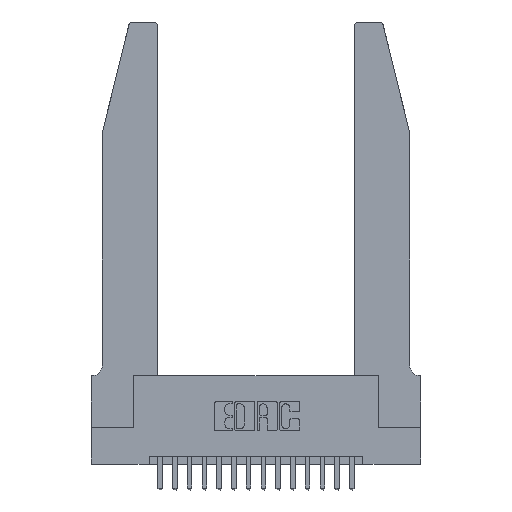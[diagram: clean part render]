
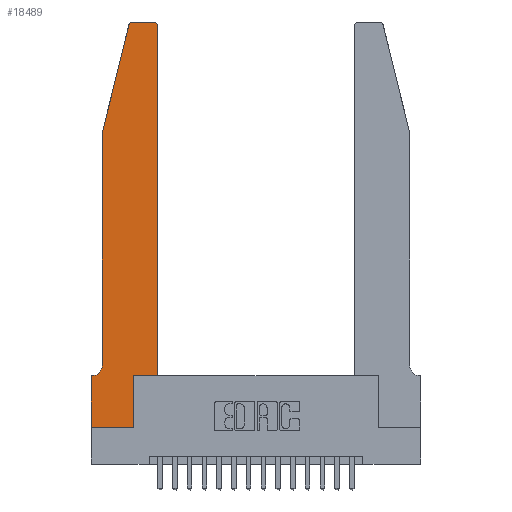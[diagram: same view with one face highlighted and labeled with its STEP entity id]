
A CAD part, top view. The second image highlights one B-rep face of the part: STEP entity #18489.
In plain terms, the highlighted planar face has unit normal (0, 0, 1).
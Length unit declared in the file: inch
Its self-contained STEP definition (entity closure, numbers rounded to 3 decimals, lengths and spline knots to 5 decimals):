
#10 = CARTESIAN_POINT ( 'NONE',  ( 0.2865, 0.35, 0.37 ) ) ;
#383 = ORIENTED_EDGE ( 'NONE', *, *, #14415, .T. ) ;
#557 = DIRECTION ( 'NONE',  ( 0., -1., 0. ) ) ;
#565 = EDGE_CURVE ( 'NONE', #1459, #2175, #1301, .T. ) ;
#657 = CARTESIAN_POINT ( 'NONE',  ( 0.25487, 2.72718, 0.37 ) ) ;
#998 = CARTESIAN_POINT ( 'NONE',  ( 0.0055, 0.35, 0.37 ) ) ;
#1287 = VERTEX_POINT ( 'NONE', #17389 ) ;
#1301 = LINE ( 'NONE', #3186, #13107 ) ;
#1307 = CARTESIAN_POINT ( 'NONE',  ( 0.284, 2.72, 0.37 ) ) ;
#1415 = DIRECTION ( 'NONE',  ( 0., 1., 0. ) ) ;
#1459 = VERTEX_POINT ( 'NONE', #657 ) ;
#1887 = ORIENTED_EDGE ( 'NONE', *, *, #7850, .T. ) ;
#1935 = LINE ( 'NONE', #6139, #17529 ) ;
#2174 = EDGE_CURVE ( 'NONE', #6548, #7849, #13315, .T. ) ;
#2175 = VERTEX_POINT ( 'NONE', #17664 ) ;
#2743 = EDGE_CURVE ( 'NONE', #13909, #16996, #7911, .T. ) ;
#2886 = LINE ( 'NONE', #12141, #7076 ) ;
#2912 = DIRECTION ( 'NONE',  ( 1., 0., 0. ) ) ;
#3186 = CARTESIAN_POINT ( 'NONE',  ( 0.0755, 2., 0.37 ) ) ;
#3540 = AXIS2_PLACEMENT_3D ( 'NONE', #13201, #4054, #14650 ) ;
#3623 = EDGE_CURVE ( 'NONE', #14515, #13909, #11487, .T. ) ;
#3735 = DIRECTION ( 'NONE',  ( 0., 0., -1. ) ) ;
#3985 = CARTESIAN_POINT ( 'NONE',  ( 0.284, 2.75, 0.37 ) ) ;
#4054 = DIRECTION ( 'NONE',  ( 0., 0., 1. ) ) ;
#4196 = VECTOR ( 'NONE', #557, 39.37008 ) ;
#4371 = VERTEX_POINT ( 'NONE', #19359 ) ;
#4675 = ORIENTED_EDGE ( 'NONE', *, *, #2743, .T. ) ;
#4690 = EDGE_CURVE ( 'NONE', #1287, #6548, #13777, .T. ) ;
#5369 = CARTESIAN_POINT ( 'NONE',  ( 0.4505, 0.35, 0.37 ) ) ;
#6056 = EDGE_CURVE ( 'NONE', #15065, #17407, #13510, .T. ) ;
#6103 = ORIENTED_EDGE ( 'NONE', *, *, #4690, .T. ) ;
#6104 = DIRECTION ( 'NONE',  ( 0., 0., 1. ) ) ;
#6133 = FACE_OUTER_BOUND ( 'NONE', #13007, .T. ) ;
#6139 = CARTESIAN_POINT ( 'NONE',  ( 0.2865, 0.35, 0.37 ) ) ;
#6401 = VERTEX_POINT ( 'NONE', #14406 ) ;
#6548 = VERTEX_POINT ( 'NONE', #998 ) ;
#6762 = CARTESIAN_POINT ( 'NONE',  ( 0.0755, 2., 0.37 ) ) ;
#7006 = ORIENTED_EDGE ( 'NONE', *, *, #2174, .T. ) ;
#7076 = VECTOR ( 'NONE', #9186, 39.37008 ) ;
#7359 = EDGE_CURVE ( 'NONE', #17407, #14515, #17080, .T. ) ;
#7425 = VECTOR ( 'NONE', #10382, 39.37008 ) ;
#7849 = VERTEX_POINT ( 'NONE', #16462 ) ;
#7850 = EDGE_CURVE ( 'NONE', #16996, #1459, #8326, .T. ) ;
#7911 = LINE ( 'NONE', #18890, #7425 ) ;
#7941 = LINE ( 'NONE', #6762, #15813 ) ;
#8326 = CIRCLE ( 'NONE', #9964, 0.03 ) ;
#8365 = LINE ( 'NONE', #12959, #4196 ) ;
#8422 = VECTOR ( 'NONE', #17616, 39.37008 ) ;
#8624 = EDGE_CURVE ( 'NONE', #4371, #6401, #2886, .T. ) ;
#9179 = AXIS2_PLACEMENT_3D ( 'NONE', #15007, #6104, #16528 ) ;
#9186 = DIRECTION ( 'NONE',  ( 1., 0., 0. ) ) ;
#9196 = ORIENTED_EDGE ( 'NONE', *, *, #17257, .T. ) ;
#9359 = CARTESIAN_POINT ( 'NONE',  ( 0.4505, 0.35, 0.37 ) ) ;
#9754 = ORIENTED_EDGE ( 'NONE', *, *, #8624, .T. ) ;
#9964 = AXIS2_PLACEMENT_3D ( 'NONE', #1307, #12104, #2912 ) ;
#10039 = VECTOR ( 'NONE', #14376, 39.37008 ) ;
#10291 = CARTESIAN_POINT ( 'NONE',  ( 0.4505, 0.35, 0.37 ) ) ;
#10382 = DIRECTION ( 'NONE',  ( -1., 0., 0. ) ) ;
#10784 = EDGE_CURVE ( 'NONE', #6401, #15065, #1935, .T. ) ;
#11259 = DIRECTION ( 'NONE',  ( 0., -1., 0. ) ) ;
#11487 = CIRCLE ( 'NONE', #3540, 0.03 ) ;
#11635 = ORIENTED_EDGE ( 'NONE', *, *, #10784, .T. ) ;
#11801 = ORIENTED_EDGE ( 'NONE', *, *, #6056, .T. ) ;
#12104 = DIRECTION ( 'NONE',  ( 0., 0., 1. ) ) ;
#12141 = CARTESIAN_POINT ( 'NONE',  ( 0., 0., 0.37 ) ) ;
#12662 = ORIENTED_EDGE ( 'NONE', *, *, #565, .T. ) ;
#12689 = ORIENTED_EDGE ( 'NONE', *, *, #7359, .T. ) ;
#12775 = ORIENTED_EDGE ( 'NONE', *, *, #3623, .T. ) ;
#12903 = CARTESIAN_POINT ( 'NONE',  ( 0.0055, 0.42, 0.37 ) ) ;
#12959 = CARTESIAN_POINT ( 'NONE',  ( 0., 0., 0.37 ) ) ;
#13007 = EDGE_LOOP ( 'NONE', ( #4675, #1887, #12662, #383, #6103, #7006, #9196, #9754, #11635, #11801, #12689, #12775 ) ) ;
#13107 = VECTOR ( 'NONE', #15917, 39.37008 ) ;
#13201 = CARTESIAN_POINT ( 'NONE',  ( 0.4205, 2.72, 0.37 ) ) ;
#13315 = LINE ( 'NONE', #17851, #8422 ) ;
#13510 = LINE ( 'NONE', #5369, #10039 ) ;
#13543 = PLANE ( 'NONE',  #9179 ) ;
#13777 = CIRCLE ( 'NONE', #16571, 0.07 ) ;
#13909 = VERTEX_POINT ( 'NONE', #16830 ) ;
#14361 = DIRECTION ( 'NONE',  ( -1., 0., 0. ) ) ;
#14376 = DIRECTION ( 'NONE',  ( 1., 0., 0. ) ) ;
#14406 = CARTESIAN_POINT ( 'NONE',  ( 0.2865, 0., 0.37 ) ) ;
#14415 = EDGE_CURVE ( 'NONE', #2175, #1287, #7941, .T. ) ;
#14515 = VERTEX_POINT ( 'NONE', #15258 ) ;
#14650 = DIRECTION ( 'NONE',  ( 1., 0., 0. ) ) ;
#15007 = CARTESIAN_POINT ( 'NONE',  ( 0., 0.35, 0.37 ) ) ;
#15065 = VERTEX_POINT ( 'NONE', #10 ) ;
#15258 = CARTESIAN_POINT ( 'NONE',  ( 0.4505, 2.72, 0.37 ) ) ;
#15729 = VECTOR ( 'NONE', #16670, 39.37008 ) ;
#15813 = VECTOR ( 'NONE', #11259, 39.37008 ) ;
#15917 = DIRECTION ( 'NONE',  ( -0.239, -0.971, 0. ) ) ;
#16462 = CARTESIAN_POINT ( 'NONE',  ( 0., 0.35, 0.37 ) ) ;
#16528 = DIRECTION ( 'NONE',  ( 1., 0., 0. ) ) ;
#16571 = AXIS2_PLACEMENT_3D ( 'NONE', #12903, #3735, #14361 ) ;
#16670 = DIRECTION ( 'NONE',  ( 0., 1., 0. ) ) ;
#16830 = CARTESIAN_POINT ( 'NONE',  ( 0.4205, 2.75, 0.37 ) ) ;
#16996 = VERTEX_POINT ( 'NONE', #3985 ) ;
#17080 = LINE ( 'NONE', #9359, #15729 ) ;
#17257 = EDGE_CURVE ( 'NONE', #7849, #4371, #8365, .T. ) ;
#17389 = CARTESIAN_POINT ( 'NONE',  ( 0.0755, 0.42, 0.37 ) ) ;
#17407 = VERTEX_POINT ( 'NONE', #10291 ) ;
#17529 = VECTOR ( 'NONE', #1415, 39.37008 ) ;
#17616 = DIRECTION ( 'NONE',  ( -1., 0., 0. ) ) ;
#17664 = CARTESIAN_POINT ( 'NONE',  ( 0.0755, 2., 0.37 ) ) ;
#17851 = CARTESIAN_POINT ( 'NONE',  ( 0.0755, 0.35, 0.37 ) ) ;
#18489 = ADVANCED_FACE ( 'NONE', ( #6133 ), #13543, .T. ) ;
#18890 = CARTESIAN_POINT ( 'NONE',  ( 0.2605, 2.75, 0.37 ) ) ;
#19359 = CARTESIAN_POINT ( 'NONE',  ( 0., 0., 0.37 ) ) ;
